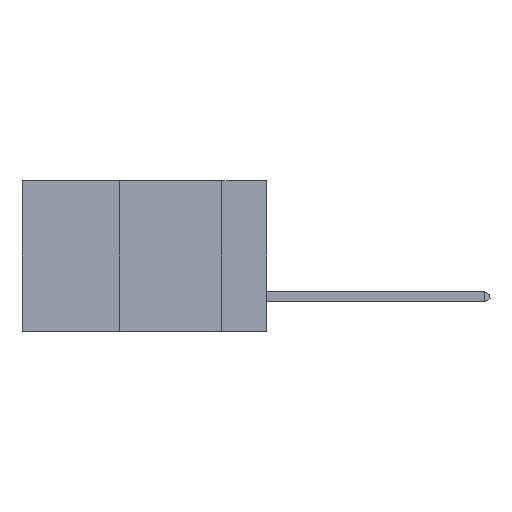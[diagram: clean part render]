
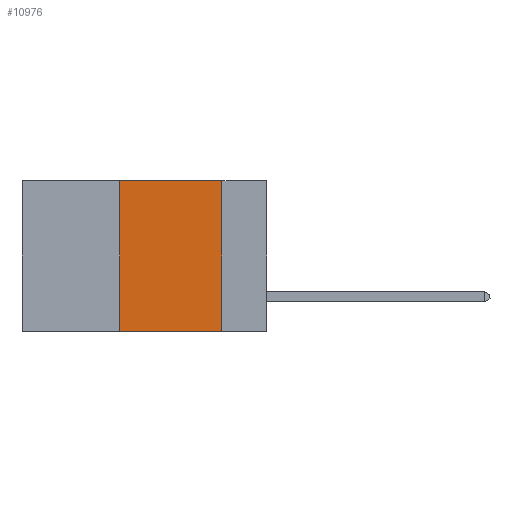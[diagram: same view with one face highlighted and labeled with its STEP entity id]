
A CAD part, left-side view. The second image highlights one B-rep face of the part: STEP entity #10976.
In plain terms, the highlighted planar face has unit normal (-1, 0, 0).
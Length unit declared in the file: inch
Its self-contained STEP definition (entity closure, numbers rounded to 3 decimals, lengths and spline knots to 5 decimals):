
#89 = ORIENTED_EDGE ( 'NONE', *, *, #8639, .F. ) ;
#130 = EDGE_CURVE ( 'NONE', #4432, #11793, #3563, .T. ) ;
#233 = CARTESIAN_POINT ( 'NONE',  ( 0., 0.36, 0. ) ) ;
#953 = LINE ( 'NONE', #12184, #3768 ) ;
#995 = CARTESIAN_POINT ( 'NONE',  ( 0., 0.11, 0. ) ) ;
#1199 = ORIENTED_EDGE ( 'NONE', *, *, #130, .F. ) ;
#1978 = DIRECTION ( 'NONE',  ( 0., -1., 0. ) ) ;
#2097 = AXIS2_PLACEMENT_3D ( 'NONE', #12326, #10222, #7054 ) ;
#2261 = DIRECTION ( 'NONE',  ( 0., -1., 0. ) ) ;
#2818 = LINE ( 'NONE', #7650, #11034 ) ;
#3490 = VECTOR ( 'NONE', #4333, 39.37008 ) ;
#3563 = LINE ( 'NONE', #10565, #11791 ) ;
#3751 = ORIENTED_EDGE ( 'NONE', *, *, #11388, .F. ) ;
#3762 = ORIENTED_EDGE ( 'NONE', *, *, #13150, .T. ) ;
#3768 = VECTOR ( 'NONE', #5764, 39.37008 ) ;
#4333 = DIRECTION ( 'NONE',  ( 0., 0., -1. ) ) ;
#4432 = VERTEX_POINT ( 'NONE', #233 ) ;
#4503 = LINE ( 'NONE', #995, #3490 ) ;
#4902 = PLANE ( 'NONE',  #2097 ) ;
#4941 = EDGE_LOOP ( 'NONE', ( #3751, #1199, #89, #3762 ) ) ;
#5764 = DIRECTION ( 'NONE',  ( 0., 0., 1. ) ) ;
#7054 = DIRECTION ( 'NONE',  ( 0., 0., -1. ) ) ;
#7650 = CARTESIAN_POINT ( 'NONE',  ( 0., 0.6, -0.37 ) ) ;
#8635 = VERTEX_POINT ( 'NONE', #8914 ) ;
#8639 = EDGE_CURVE ( 'NONE', #8635, #4432, #953, .T. ) ;
#8914 = CARTESIAN_POINT ( 'NONE',  ( 0., 0.36, -0.37 ) ) ;
#10128 = CARTESIAN_POINT ( 'NONE',  ( 0., 0.11, -0.37 ) ) ;
#10222 = DIRECTION ( 'NONE',  ( 1., 0., 0. ) ) ;
#10565 = CARTESIAN_POINT ( 'NONE',  ( 0., 0.6, 0. ) ) ;
#10976 = ADVANCED_FACE ( 'NONE', ( #13107 ), #4902, .F. ) ;
#11034 = VECTOR ( 'NONE', #2261, 39.37008 ) ;
#11388 = EDGE_CURVE ( 'NONE', #11793, #11637, #4503, .T. ) ;
#11637 = VERTEX_POINT ( 'NONE', #10128 ) ;
#11791 = VECTOR ( 'NONE', #1978, 39.37008 ) ;
#11793 = VERTEX_POINT ( 'NONE', #13747 ) ;
#12184 = CARTESIAN_POINT ( 'NONE',  ( 0., 0.36, 0. ) ) ;
#12326 = CARTESIAN_POINT ( 'NONE',  ( 0., 0.6, 0. ) ) ;
#13107 = FACE_OUTER_BOUND ( 'NONE', #4941, .T. ) ;
#13150 = EDGE_CURVE ( 'NONE', #8635, #11637, #2818, .T. ) ;
#13747 = CARTESIAN_POINT ( 'NONE',  ( 0., 0.11, 0. ) ) ;
